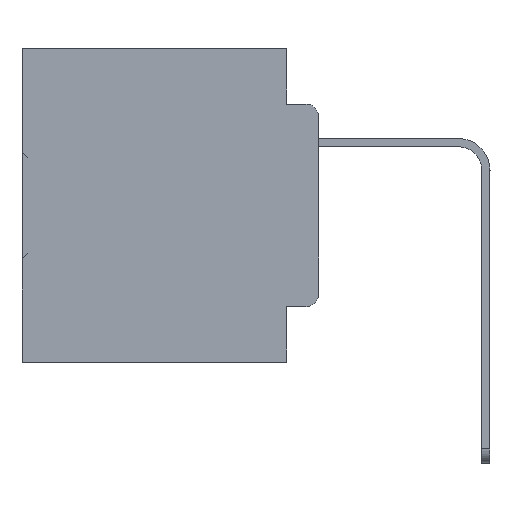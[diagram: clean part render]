
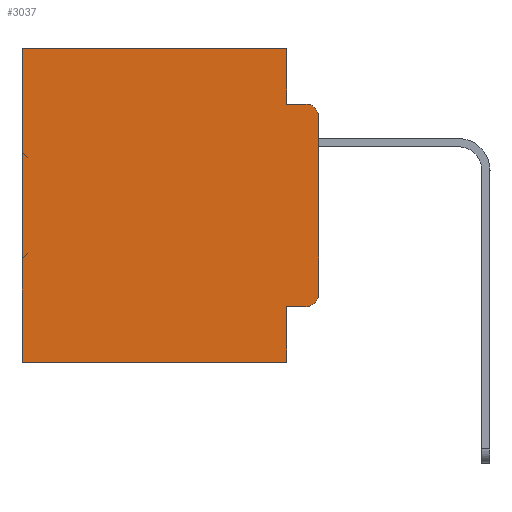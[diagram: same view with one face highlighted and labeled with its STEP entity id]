
A CAD part, left-side view. The second image highlights one B-rep face of the part: STEP entity #3037.
In plain terms, the highlighted planar face has unit normal (-1, 0, 0).
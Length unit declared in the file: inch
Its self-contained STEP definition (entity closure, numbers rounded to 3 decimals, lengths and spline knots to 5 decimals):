
#315 = CARTESIAN_POINT ( 'NONE',  ( 0.298, 0.051, -0.0885 ) ) ;
#381 = CARTESIAN_POINT ( 'NONE',  ( 0.298, 0., 0. ) ) ;
#732 = CIRCLE ( 'NONE', #6245, 0.02 ) ;
#1805 = CARTESIAN_POINT ( 'NONE',  ( 0.298, 0., 0. ) ) ;
#2415 = VERTEX_POINT ( 'NONE', #7383 ) ;
#2464 = CARTESIAN_POINT ( 'NONE',  ( 0.298, 0.02, -0.4115 ) ) ;
#2788 = DIRECTION ( 'NONE',  ( 0., 0., -1. ) ) ;
#2900 = CARTESIAN_POINT ( 'NONE',  ( 0.298, 0.02, -0.1085 ) ) ;
#3037 = ADVANCED_FACE ( 'NONE', ( #35142 ), #19617, .F. ) ;
#4001 = LINE ( 'NONE', #315, #9780 ) ;
#4318 = VERTEX_POINT ( 'NONE', #2464 ) ;
#4330 = ORIENTED_EDGE ( 'NONE', *, *, #20335, .F. ) ;
#5012 = LINE ( 'NONE', #34524, #7272 ) ;
#5063 = CARTESIAN_POINT ( 'NONE',  ( 0.298, 0., 0. ) ) ;
#5358 = EDGE_LOOP ( 'NONE', ( #35031, #22473, #4330, #16164, #14354, #19807, #10631, #16222, #18014, #15031 ) ) ;
#5451 = DIRECTION ( 'NONE',  ( 0., -1., 0. ) ) ;
#5573 = CARTESIAN_POINT ( 'NONE',  ( 0.298, 0.473, 0. ) ) ;
#5722 = VECTOR ( 'NONE', #20437, 39.37008 ) ;
#6211 = DIRECTION ( 'NONE',  ( 0., 1., 0. ) ) ;
#6245 = AXIS2_PLACEMENT_3D ( 'NONE', #2900, #37261, #2788 ) ;
#7115 = EDGE_CURVE ( 'NONE', #33335, #22114, #8716, .T. ) ;
#7272 = VECTOR ( 'NONE', #31610, 39.37008 ) ;
#7374 = DIRECTION ( 'NONE',  ( -1., 0., 0. ) ) ;
#7383 = CARTESIAN_POINT ( 'NONE',  ( 0.298, 0.473, 0. ) ) ;
#7417 = CARTESIAN_POINT ( 'NONE',  ( 0.298, 0.051, -0.5 ) ) ;
#7776 = CARTESIAN_POINT ( 'NONE',  ( 0.298, 0., -0.1085 ) ) ;
#8407 = VERTEX_POINT ( 'NONE', #33895 ) ;
#8592 = LINE ( 'NONE', #1805, #25676 ) ;
#8701 = CARTESIAN_POINT ( 'NONE',  ( 0.298, 0.473, -0.5 ) ) ;
#8716 = LINE ( 'NONE', #32295, #23584 ) ;
#9220 = EDGE_CURVE ( 'NONE', #2415, #15437, #31974, .T. ) ;
#9780 = VECTOR ( 'NONE', #5451, 39.37008 ) ;
#10631 = ORIENTED_EDGE ( 'NONE', *, *, #34200, .F. ) ;
#11133 = DIRECTION ( 'NONE',  ( 0., 0., -1. ) ) ;
#11553 = LINE ( 'NONE', #381, #5722 ) ;
#11564 = DIRECTION ( 'NONE',  ( 0., -1., 0. ) ) ;
#13745 = EDGE_CURVE ( 'NONE', #32211, #26509, #5012, .T. ) ;
#13920 = CIRCLE ( 'NONE', #15715, 0.02 ) ;
#14275 = AXIS2_PLACEMENT_3D ( 'NONE', #5063, #28053, #16362 ) ;
#14354 = ORIENTED_EDGE ( 'NONE', *, *, #28795, .T. ) ;
#15031 = ORIENTED_EDGE ( 'NONE', *, *, #27068, .T. ) ;
#15437 = VERTEX_POINT ( 'NONE', #8701 ) ;
#15715 = AXIS2_PLACEMENT_3D ( 'NONE', #18558, #7374, #33052 ) ;
#16164 = ORIENTED_EDGE ( 'NONE', *, *, #7115, .F. ) ;
#16222 = ORIENTED_EDGE ( 'NONE', *, *, #13745, .F. ) ;
#16362 = DIRECTION ( 'NONE',  ( 0., 0., -1. ) ) ;
#16547 = CARTESIAN_POINT ( 'NONE',  ( 0.298, 0.051, -0.4115 ) ) ;
#16811 = VECTOR ( 'NONE', #11564, 39.37008 ) ;
#18014 = ORIENTED_EDGE ( 'NONE', *, *, #24642, .T. ) ;
#18558 = CARTESIAN_POINT ( 'NONE',  ( 0.298, 0.02, -0.3915 ) ) ;
#19213 = DIRECTION ( 'NONE',  ( 0., 0., -1. ) ) ;
#19617 = PLANE ( 'NONE',  #14275 ) ;
#19625 = CARTESIAN_POINT ( 'NONE',  ( 0.298, 0.02, -0.0885 ) ) ;
#19807 = ORIENTED_EDGE ( 'NONE', *, *, #9220, .T. ) ;
#20335 = EDGE_CURVE ( 'NONE', #22114, #27913, #4001, .T. ) ;
#20437 = DIRECTION ( 'NONE',  ( 0., 1., 0. ) ) ;
#22114 = VERTEX_POINT ( 'NONE', #31034 ) ;
#22473 = ORIENTED_EDGE ( 'NONE', *, *, #33501, .T. ) ;
#22627 = CARTESIAN_POINT ( 'NONE',  ( 0.298, 0.051, -0.4115 ) ) ;
#23405 = VECTOR ( 'NONE', #25657, 39.37008 ) ;
#23584 = VECTOR ( 'NONE', #11133, 39.37008 ) ;
#24642 = EDGE_CURVE ( 'NONE', #32211, #4318, #27608, .T. ) ;
#25657 = DIRECTION ( 'NONE',  ( 0., 0., -1. ) ) ;
#25676 = VECTOR ( 'NONE', #19213, 39.37008 ) ;
#26507 = EDGE_CURVE ( 'NONE', #33435, #8407, #8592, .T. ) ;
#26509 = VERTEX_POINT ( 'NONE', #7417 ) ;
#27068 = EDGE_CURVE ( 'NONE', #4318, #8407, #13920, .T. ) ;
#27608 = LINE ( 'NONE', #22627, #16811 ) ;
#27913 = VERTEX_POINT ( 'NONE', #19625 ) ;
#28053 = DIRECTION ( 'NONE',  ( 1., 0., 0. ) ) ;
#28084 = VECTOR ( 'NONE', #6211, 39.37008 ) ;
#28795 = EDGE_CURVE ( 'NONE', #33335, #2415, #11553, .T. ) ;
#29452 = LINE ( 'NONE', #35425, #28084 ) ;
#30160 = CARTESIAN_POINT ( 'NONE',  ( 0.298, 0.051, 0. ) ) ;
#31034 = CARTESIAN_POINT ( 'NONE',  ( 0.298, 0.051, -0.0885 ) ) ;
#31610 = DIRECTION ( 'NONE',  ( 0., 0., -1. ) ) ;
#31974 = LINE ( 'NONE', #5573, #23405 ) ;
#32211 = VERTEX_POINT ( 'NONE', #16547 ) ;
#32295 = CARTESIAN_POINT ( 'NONE',  ( 0.298, 0.051, 0. ) ) ;
#33052 = DIRECTION ( 'NONE',  ( 0., 0., -1. ) ) ;
#33335 = VERTEX_POINT ( 'NONE', #30160 ) ;
#33435 = VERTEX_POINT ( 'NONE', #7776 ) ;
#33501 = EDGE_CURVE ( 'NONE', #33435, #27913, #732, .T. ) ;
#33895 = CARTESIAN_POINT ( 'NONE',  ( 0.298, 0., -0.3915 ) ) ;
#34200 = EDGE_CURVE ( 'NONE', #26509, #15437, #29452, .T. ) ;
#34524 = CARTESIAN_POINT ( 'NONE',  ( 0.298, 0.051, 0. ) ) ;
#35031 = ORIENTED_EDGE ( 'NONE', *, *, #26507, .F. ) ;
#35142 = FACE_OUTER_BOUND ( 'NONE', #5358, .T. ) ;
#35425 = CARTESIAN_POINT ( 'NONE',  ( 0.298, 0., -0.5 ) ) ;
#37261 = DIRECTION ( 'NONE',  ( -1., 0., 0. ) ) ;
